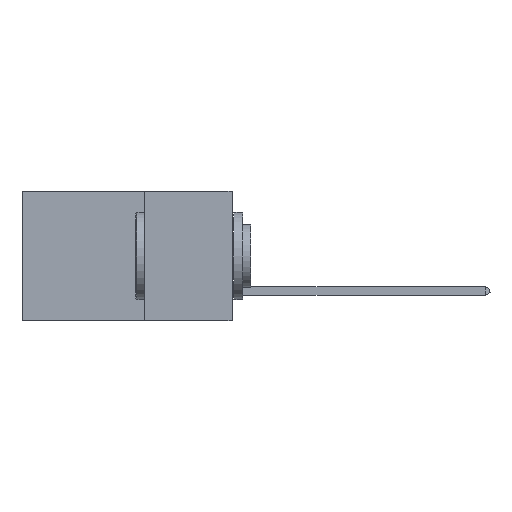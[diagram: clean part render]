
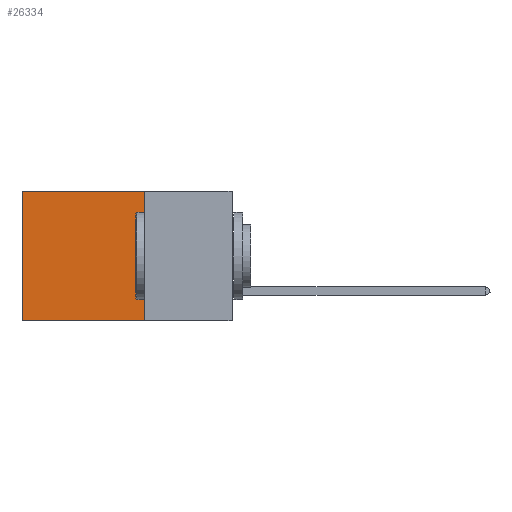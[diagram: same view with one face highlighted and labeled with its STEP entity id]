
A CAD part, left-side view. The second image highlights one B-rep face of the part: STEP entity #26334.
In plain terms, the highlighted planar face has unit normal (-1, 0, 0).
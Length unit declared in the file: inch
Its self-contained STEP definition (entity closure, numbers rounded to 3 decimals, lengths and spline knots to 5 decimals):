
#2159 = CARTESIAN_POINT ( 'NONE',  ( 0.2875, 0.25, -0.37 ) ) ;
#2320 = CARTESIAN_POINT ( 'NONE',  ( 0.2875, 0.25, 0. ) ) ;
#4291 = VECTOR ( 'NONE', #16132, 39.37008 ) ;
#5286 = EDGE_CURVE ( 'NONE', #11602, #35781, #38089, .T. ) ;
#7314 = ORIENTED_EDGE ( 'NONE', *, *, #5286, .F. ) ;
#8232 = AXIS2_PLACEMENT_3D ( 'NONE', #27305, #20093, #34521 ) ;
#10095 = LINE ( 'NONE', #45412, #4291 ) ;
#10137 = VERTEX_POINT ( 'NONE', #28247 ) ;
#10548 = EDGE_CURVE ( 'NONE', #11602, #10137, #34698, .T. ) ;
#11155 = EDGE_CURVE ( 'NONE', #35781, #32072, #17479, .T. ) ;
#11602 = VERTEX_POINT ( 'NONE', #47680 ) ;
#12140 = CARTESIAN_POINT ( 'NONE',  ( 0.2875, 0.25, -0.37 ) ) ;
#13988 = EDGE_LOOP ( 'NONE', ( #47589, #44610, #7314, #20239 ) ) ;
#16095 = CARTESIAN_POINT ( 'NONE',  ( 0.2875, 0.25, 0. ) ) ;
#16132 = DIRECTION ( 'NONE',  ( 0., 0., -1. ) ) ;
#16558 = DIRECTION ( 'NONE',  ( 0., 1., 0. ) ) ;
#16855 = DIRECTION ( 'NONE',  ( 0., 0., -1. ) ) ;
#17479 = LINE ( 'NONE', #12140, #44514 ) ;
#20093 = DIRECTION ( 'NONE',  ( 1., 0., 0. ) ) ;
#20239 = ORIENTED_EDGE ( 'NONE', *, *, #10548, .T. ) ;
#24926 = VECTOR ( 'NONE', #16558, 39.37008 ) ;
#26334 = ADVANCED_FACE ( 'NONE', ( #46027 ), #45959, .F. ) ;
#27305 = CARTESIAN_POINT ( 'NONE',  ( 0.2875, 0.25, 0. ) ) ;
#28247 = CARTESIAN_POINT ( 'NONE',  ( 0.2875, 0.6, 0. ) ) ;
#31141 = EDGE_CURVE ( 'NONE', #10137, #32072, #10095, .T. ) ;
#32072 = VERTEX_POINT ( 'NONE', #35996 ) ;
#34366 = DIRECTION ( 'NONE',  ( 0., 1., 0. ) ) ;
#34521 = DIRECTION ( 'NONE',  ( 0., 0., -1. ) ) ;
#34698 = LINE ( 'NONE', #16095, #24926 ) ;
#35781 = VERTEX_POINT ( 'NONE', #2159 ) ;
#35996 = CARTESIAN_POINT ( 'NONE',  ( 0.2875, 0.6, -0.37 ) ) ;
#36926 = VECTOR ( 'NONE', #16855, 39.37008 ) ;
#38089 = LINE ( 'NONE', #2320, #36926 ) ;
#44514 = VECTOR ( 'NONE', #34366, 39.37008 ) ;
#44610 = ORIENTED_EDGE ( 'NONE', *, *, #11155, .F. ) ;
#45412 = CARTESIAN_POINT ( 'NONE',  ( 0.2875, 0.6, 0. ) ) ;
#45959 = PLANE ( 'NONE',  #8232 ) ;
#46027 = FACE_OUTER_BOUND ( 'NONE', #13988, .T. ) ;
#47589 = ORIENTED_EDGE ( 'NONE', *, *, #31141, .T. ) ;
#47680 = CARTESIAN_POINT ( 'NONE',  ( 0.2875, 0.25, 0. ) ) ;
